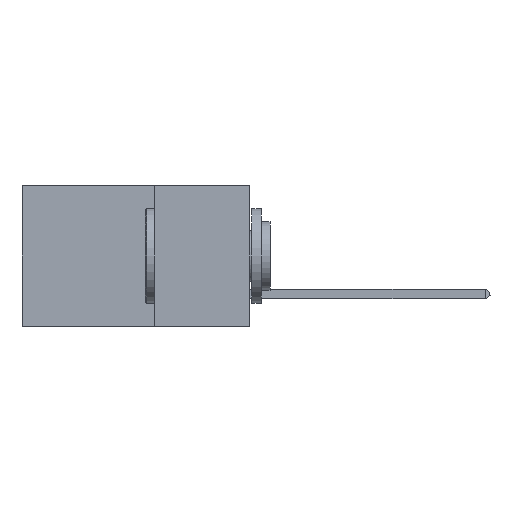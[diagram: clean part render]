
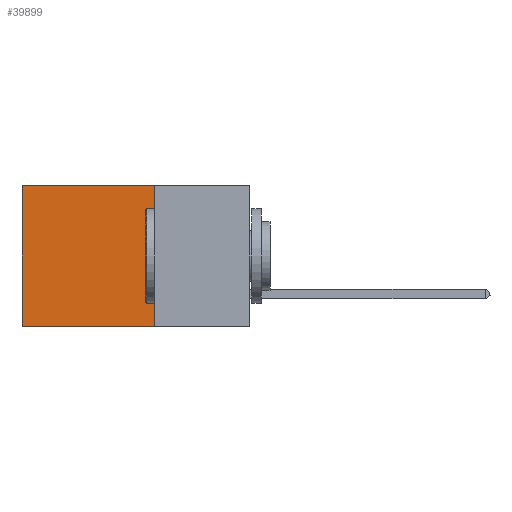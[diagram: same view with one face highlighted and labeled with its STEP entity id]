
A CAD part, left-side view. The second image highlights one B-rep face of the part: STEP entity #39899.
In plain terms, the highlighted planar face has unit normal (-1, 0, 0).
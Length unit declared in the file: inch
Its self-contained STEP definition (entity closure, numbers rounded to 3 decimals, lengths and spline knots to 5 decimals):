
#1405 = VERTEX_POINT ( 'NONE', #42273 ) ;
#2444 = DIRECTION ( 'NONE',  ( 1., 0., 0. ) ) ;
#3621 = LINE ( 'NONE', #22313, #19402 ) ;
#5361 = VERTEX_POINT ( 'NONE', #9614 ) ;
#5673 = CARTESIAN_POINT ( 'NONE',  ( 0.2875, 0.6, 0. ) ) ;
#5694 = EDGE_CURVE ( 'NONE', #5361, #36097, #3621, .T. ) ;
#5838 = AXIS2_PLACEMENT_3D ( 'NONE', #41429, #2444, #15363 ) ;
#8769 = ORIENTED_EDGE ( 'NONE', *, *, #34624, .T. ) ;
#9280 = DIRECTION ( 'NONE',  ( 0., 1., 0. ) ) ;
#9614 = CARTESIAN_POINT ( 'NONE',  ( 0.2875, 0.25, 0. ) ) ;
#9796 = VERTEX_POINT ( 'NONE', #19440 ) ;
#14053 = ORIENTED_EDGE ( 'NONE', *, *, #34430, .F. ) ;
#15363 = DIRECTION ( 'NONE',  ( 0., 0., -1. ) ) ;
#17667 = LINE ( 'NONE', #31435, #36546 ) ;
#17723 = FACE_OUTER_BOUND ( 'NONE', #42890, .T. ) ;
#19402 = VECTOR ( 'NONE', #9280, 39.37008 ) ;
#19440 = CARTESIAN_POINT ( 'NONE',  ( 0.2875, 0.6, -0.37 ) ) ;
#20803 = VECTOR ( 'NONE', #37430, 39.37008 ) ;
#22313 = CARTESIAN_POINT ( 'NONE',  ( 0.2875, 0.25, 0. ) ) ;
#22541 = DIRECTION ( 'NONE',  ( 0., 0., -1. ) ) ;
#26910 = CARTESIAN_POINT ( 'NONE',  ( 0.2875, 0.25, 0. ) ) ;
#28650 = PLANE ( 'NONE',  #5838 ) ;
#29373 = CARTESIAN_POINT ( 'NONE',  ( 0.2875, 0.6, 0. ) ) ;
#30315 = EDGE_CURVE ( 'NONE', #5361, #1405, #35024, .T. ) ;
#31435 = CARTESIAN_POINT ( 'NONE',  ( 0.2875, 0.25, -0.37 ) ) ;
#32321 = ORIENTED_EDGE ( 'NONE', *, *, #30315, .F. ) ;
#33917 = VECTOR ( 'NONE', #22541, 39.37008 ) ;
#34430 = EDGE_CURVE ( 'NONE', #1405, #9796, #17667, .T. ) ;
#34624 = EDGE_CURVE ( 'NONE', #36097, #9796, #37063, .T. ) ;
#35024 = LINE ( 'NONE', #26910, #20803 ) ;
#36097 = VERTEX_POINT ( 'NONE', #29373 ) ;
#36546 = VECTOR ( 'NONE', #41310, 39.37008 ) ;
#37063 = LINE ( 'NONE', #5673, #33917 ) ;
#37215 = ORIENTED_EDGE ( 'NONE', *, *, #5694, .T. ) ;
#37430 = DIRECTION ( 'NONE',  ( 0., 0., -1. ) ) ;
#39899 = ADVANCED_FACE ( 'NONE', ( #17723 ), #28650, .F. ) ;
#41310 = DIRECTION ( 'NONE',  ( 0., 1., 0. ) ) ;
#41429 = CARTESIAN_POINT ( 'NONE',  ( 0.2875, 0.25, 0. ) ) ;
#42273 = CARTESIAN_POINT ( 'NONE',  ( 0.2875, 0.25, -0.37 ) ) ;
#42890 = EDGE_LOOP ( 'NONE', ( #8769, #14053, #32321, #37215 ) ) ;
